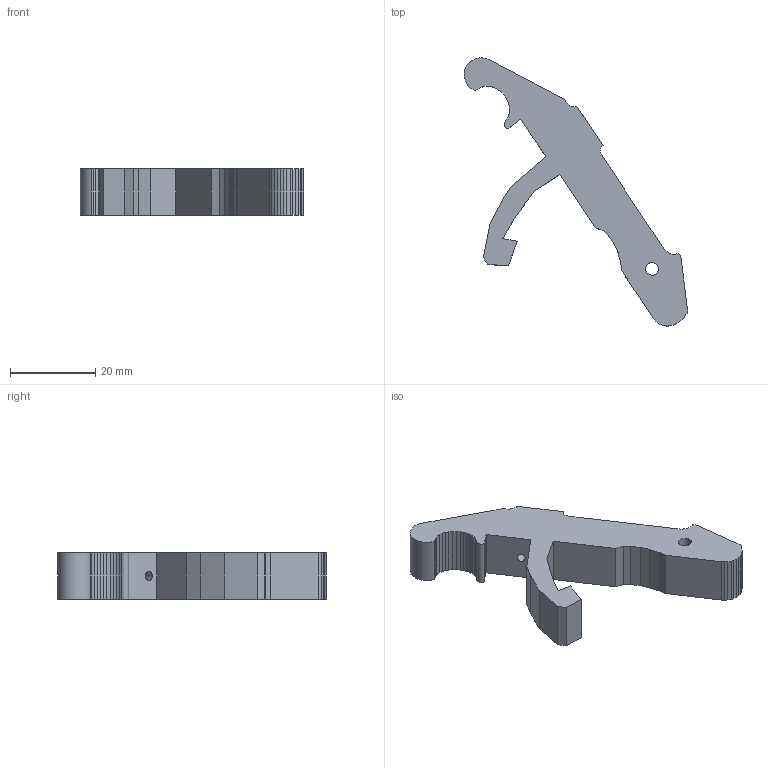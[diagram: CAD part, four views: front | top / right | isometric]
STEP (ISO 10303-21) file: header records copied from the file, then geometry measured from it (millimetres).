
FILE_DESCRIPTION((''),'2;1');
FILE_NAME('hammer.stp','2013-07-01T18:24:22',('mrfr'),(''),'Autodesk Inventor 2013','Autodesk Inventor 2013','');
FILE_SCHEMA(('AUTOMOTIVE_DESIGN { 1 0 10303 214 1 1 1 1 }'));
Length unit declared in the file: millimetre
Products named in the file (1): derringer_spoust
Bounding box: 52.44 x 62.95 x 11 mm (x, y, z)
Volume: 10189.8 mm3; surface area: 4703.6 mm2
Topology: 1 solids, 1 shells, 90 faces, 264 edges, 176 vertices
Faces by surface type: plane 86, cylinder 4
Full cylindrical faces by diameter (mm): 2 x1, 3 x1
Entity records: 2960 total; most frequent: CARTESIAN_POINT 529, ORIENTED_EDGE 524, DIRECTION 452, EDGE_CURVE 262, VECTOR 254, LINE 254, VERTEX_POINT 176, AXIS2_PLACEMENT_3D 99
